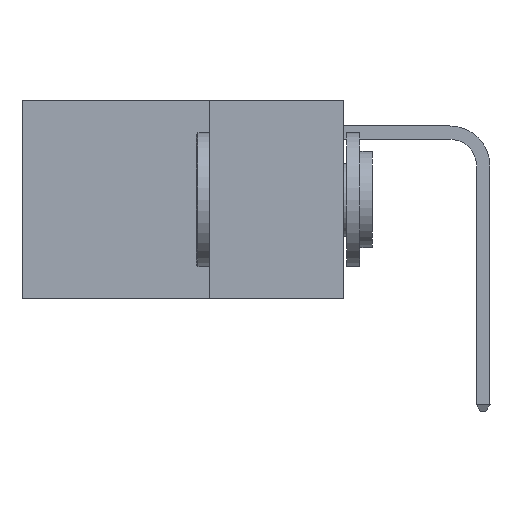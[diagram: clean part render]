
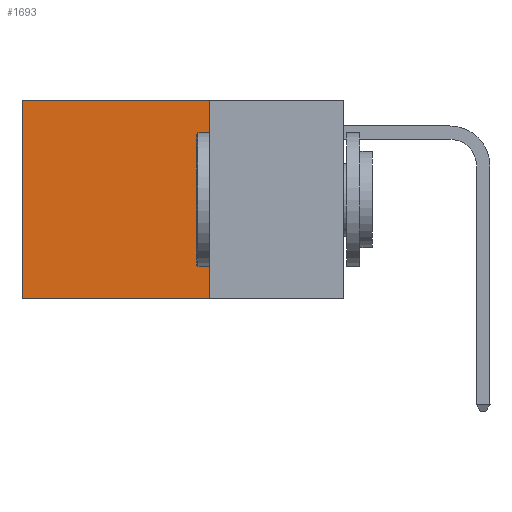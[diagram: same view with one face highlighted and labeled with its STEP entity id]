
A CAD part, left-side view. The second image highlights one B-rep face of the part: STEP entity #1693.
In plain terms, the highlighted planar face has unit normal (-1, 0, 0).
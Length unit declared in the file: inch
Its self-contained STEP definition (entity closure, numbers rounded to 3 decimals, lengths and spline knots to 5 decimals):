
#316 = EDGE_CURVE ( 'NONE', #1850, #22460, #6421, .T. ) ;
#323 = VERTEX_POINT ( 'NONE', #21100 ) ;
#1040 = FACE_OUTER_BOUND ( 'NONE', #15336, .T. ) ;
#1693 = ADVANCED_FACE ( 'NONE', ( #1040 ), #3037, .F. ) ;
#1850 = VERTEX_POINT ( 'NONE', #16546 ) ;
#2211 = CARTESIAN_POINT ( 'NONE',  ( 0.2625, 0.6, -0.37 ) ) ;
#3037 = PLANE ( 'NONE',  #16401 ) ;
#3065 = DIRECTION ( 'NONE',  ( 0., 1., 0. ) ) ;
#3178 = DIRECTION ( 'NONE',  ( 1., 0., 0. ) ) ;
#3220 = ORIENTED_EDGE ( 'NONE', *, *, #18731, .F. ) ;
#3225 = CARTESIAN_POINT ( 'NONE',  ( 0.2625, 0.6, 0. ) ) ;
#3247 = EDGE_CURVE ( 'NONE', #17127, #22460, #24730, .T. ) ;
#4151 = ORIENTED_EDGE ( 'NONE', *, *, #316, .F. ) ;
#6421 = LINE ( 'NONE', #19526, #10096 ) ;
#7036 = LINE ( 'NONE', #22253, #15031 ) ;
#10096 = VECTOR ( 'NONE', #3065, 39.37008 ) ;
#11443 = DIRECTION ( 'NONE',  ( 0., 0., -1. ) ) ;
#11516 = LINE ( 'NONE', #20479, #14129 ) ;
#11855 = DIRECTION ( 'NONE',  ( 0., 0., -1. ) ) ;
#11902 = DIRECTION ( 'NONE',  ( 0., 0., -1. ) ) ;
#13968 = CARTESIAN_POINT ( 'NONE',  ( 0.2625, 0.25, 0. ) ) ;
#14129 = VECTOR ( 'NONE', #20214, 39.37008 ) ;
#15031 = VECTOR ( 'NONE', #11443, 39.37008 ) ;
#15336 = EDGE_LOOP ( 'NONE', ( #18716, #4151, #3220, #22916 ) ) ;
#16401 = AXIS2_PLACEMENT_3D ( 'NONE', #13968, #3178, #11855 ) ;
#16546 = CARTESIAN_POINT ( 'NONE',  ( 0.2625, 0.25, -0.37 ) ) ;
#17127 = VERTEX_POINT ( 'NONE', #23417 ) ;
#18716 = ORIENTED_EDGE ( 'NONE', *, *, #3247, .T. ) ;
#18731 = EDGE_CURVE ( 'NONE', #323, #1850, #7036, .T. ) ;
#19526 = CARTESIAN_POINT ( 'NONE',  ( 0.2625, 0.25, -0.37 ) ) ;
#20214 = DIRECTION ( 'NONE',  ( 0., 1., 0. ) ) ;
#20479 = CARTESIAN_POINT ( 'NONE',  ( 0.2625, 0.25, 0. ) ) ;
#21100 = CARTESIAN_POINT ( 'NONE',  ( 0.2625, 0.25, 0. ) ) ;
#21571 = VECTOR ( 'NONE', #11902, 39.37008 ) ;
#22253 = CARTESIAN_POINT ( 'NONE',  ( 0.2625, 0.25, 0. ) ) ;
#22460 = VERTEX_POINT ( 'NONE', #2211 ) ;
#22916 = ORIENTED_EDGE ( 'NONE', *, *, #27931, .T. ) ;
#23417 = CARTESIAN_POINT ( 'NONE',  ( 0.2625, 0.6, 0. ) ) ;
#24730 = LINE ( 'NONE', #3225, #21571 ) ;
#27931 = EDGE_CURVE ( 'NONE', #323, #17127, #11516, .T. ) ;
